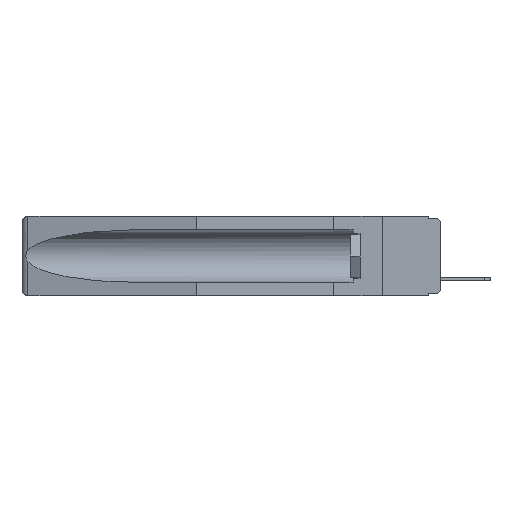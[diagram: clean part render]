
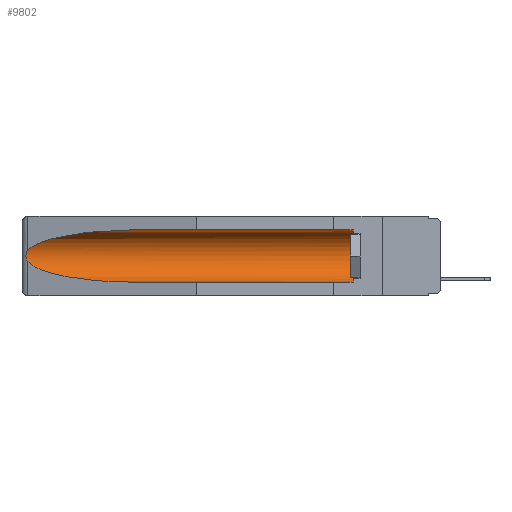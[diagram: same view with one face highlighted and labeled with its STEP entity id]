
A CAD part, left-side view. The second image highlights one B-rep face of the part: STEP entity #9802.
In plain terms, the highlighted cylindrical face has radius 2.857 mm (diameter 5.715 mm), a partial arc.
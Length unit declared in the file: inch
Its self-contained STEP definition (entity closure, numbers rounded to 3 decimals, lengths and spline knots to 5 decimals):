
#357 = VECTOR ( 'NONE', #11340, 39.37008 ) ;
#652 = ORIENTED_EDGE ( 'NONE', *, *, #13948, .F. ) ;
#1512 = CARTESIAN_POINT ( 'NONE',  ( 0.26655, 1.53094, -0.18657 ) ) ;
#1581 = B_SPLINE_CURVE_WITH_KNOTS ( 'NONE', 3,
 ( #2732, #9397, #1680, #13394, #14786, #6887, #8199, #1512, #14873, #12011 ),
 .UNSPECIFIED., .F., .F.,
 ( 4, 2, 2, 2, 4 ),
 ( 0., 0.00029, 0.00058, 0.00087, 0.00117 ),
 .UNSPECIFIED. ) ;
#1680 = CARTESIAN_POINT ( 'NONE',  ( 0.26654, 1.53092, -0.15636 ) ) ;
#2118 = EDGE_CURVE ( 'NONE', #3952, #15262, #4069, .T. ) ;
#2311 = CARTESIAN_POINT ( 'NONE',  ( 0.155, 0.126, -0.1715 ) ) ;
#2732 = CARTESIAN_POINT ( 'NONE',  ( 0.26537, 1.52718, -0.14972 ) ) ;
#3671 = VERTEX_POINT ( 'NONE', #10813 ) ;
#3677 = ORIENTED_EDGE ( 'NONE', *, *, #16923, .T. ) ;
#3952 = VERTEX_POINT ( 'NONE', #11153 ) ;
#4069 =( BOUNDED_CURVE ( )  B_SPLINE_CURVE ( 3, ( #6143, #15267, #11444, #15355 ),
 .UNSPECIFIED., .F., .T. ) 
 B_SPLINE_CURVE_WITH_KNOTS ( ( 4, 4 ),
 ( 0.1948, 1.5708 ),
 .UNSPECIFIED. ) 
 CURVE ( )  GEOMETRIC_REPRESENTATION_ITEM ( )  RATIONAL_B_SPLINE_CURVE ( ( 1., 0.848, 0.848, 1. ) ) 
 REPRESENTATION_ITEM ( '' )  );
#4642 = DIRECTION ( 'NONE',  ( 0., 0., 1. ) ) ;
#4895 = CARTESIAN_POINT ( 'NONE',  ( 0.155, -0.30754, -0.1715 ) ) ;
#4920 = CARTESIAN_POINT ( 'NONE',  ( 0.21114, 1.30732, -0.059 ) ) ;
#5428 =( BOUNDED_CURVE ( )  B_SPLINE_CURVE ( 3, ( #12991, #4920, #10303, #7452 ),
 .UNSPECIFIED., .F., .T. ) 
 B_SPLINE_CURVE_WITH_KNOTS ( ( 4, 4 ),
 ( 4.71239, 6.08839 ),
 .UNSPECIFIED. ) 
 CURVE ( )  GEOMETRIC_REPRESENTATION_ITEM ( )  RATIONAL_B_SPLINE_CURVE ( ( 1., 0.848, 0.848, 1. ) ) 
 REPRESENTATION_ITEM ( '' )  );
#6031 = ORIENTED_EDGE ( 'NONE', *, *, #16534, .T. ) ;
#6135 = ORIENTED_EDGE ( 'NONE', *, *, #2118, .T. ) ;
#6143 = CARTESIAN_POINT ( 'NONE',  ( 0.26537, 1.52718, -0.19328 ) ) ;
#6273 = VERTEX_POINT ( 'NONE', #8053 ) ;
#6887 = CARTESIAN_POINT ( 'NONE',  ( 0.2675, 1.53308, -0.17534 ) ) ;
#7030 = EDGE_LOOP ( 'NONE', ( #6031, #11529, #6135, #652, #3677, #14416 ) ) ;
#7452 = CARTESIAN_POINT ( 'NONE',  ( 0.26537, 1.52718, -0.14972 ) ) ;
#7503 = CARTESIAN_POINT ( 'NONE',  ( 0.155, -0.30754, -0.284 ) ) ;
#8053 = CARTESIAN_POINT ( 'NONE',  ( 0.155, 1.07973, -0.059 ) ) ;
#8199 = CARTESIAN_POINT ( 'NONE',  ( 0.2673, 1.53269, -0.17917 ) ) ;
#9397 = CARTESIAN_POINT ( 'NONE',  ( 0.26597, 1.52961, -0.15275 ) ) ;
#9802 = ADVANCED_FACE ( 'NONE', ( #11234 ), #16543, .F. ) ;
#9959 = CARTESIAN_POINT ( 'NONE',  ( 0.155, -0.30754, -0.059 ) ) ;
#10303 = CARTESIAN_POINT ( 'NONE',  ( 0.25451, 1.48313, -0.09465 ) ) ;
#10427 = VERTEX_POINT ( 'NONE', #13542 ) ;
#10813 = CARTESIAN_POINT ( 'NONE',  ( 0.155, 0.126, -0.284 ) ) ;
#11153 = CARTESIAN_POINT ( 'NONE',  ( 0.26537, 1.52718, -0.19328 ) ) ;
#11234 = FACE_OUTER_BOUND ( 'NONE', #7030, .T. ) ;
#11340 = DIRECTION ( 'NONE',  ( 0., 1., 0. ) ) ;
#11444 = CARTESIAN_POINT ( 'NONE',  ( 0.21114, 1.30732, -0.284 ) ) ;
#11529 = ORIENTED_EDGE ( 'NONE', *, *, #15424, .T. ) ;
#12011 = CARTESIAN_POINT ( 'NONE',  ( 0.26537, 1.52718, -0.19328 ) ) ;
#12796 = DIRECTION ( 'NONE',  ( 0., 1., 0. ) ) ;
#12822 = LINE ( 'NONE', #9959, #357 ) ;
#12969 = DIRECTION ( 'NONE',  ( 0., 0., 1. ) ) ;
#12991 = CARTESIAN_POINT ( 'NONE',  ( 0.155, 1.07973, -0.059 ) ) ;
#13144 = CARTESIAN_POINT ( 'NONE',  ( 0.155, 0.126, -0.059 ) ) ;
#13357 = VECTOR ( 'NONE', #12796, 39.37008 ) ;
#13394 = CARTESIAN_POINT ( 'NONE',  ( 0.2673, 1.5327, -0.16383 ) ) ;
#13542 = CARTESIAN_POINT ( 'NONE',  ( 0.26537, 1.52718, -0.14972 ) ) ;
#13948 = EDGE_CURVE ( 'NONE', #3671, #15262, #15146, .T. ) ;
#14025 = DIRECTION ( 'NONE',  ( 0., -1., 0. ) ) ;
#14416 = ORIENTED_EDGE ( 'NONE', *, *, #14694, .T. ) ;
#14470 = AXIS2_PLACEMENT_3D ( 'NONE', #4895, #15058, #4642 ) ;
#14694 = EDGE_CURVE ( 'NONE', #17107, #6273, #12822, .T. ) ;
#14786 = CARTESIAN_POINT ( 'NONE',  ( 0.2675, 1.53308, -0.16763 ) ) ;
#14873 = CARTESIAN_POINT ( 'NONE',  ( 0.26597, 1.5296, -0.19026 ) ) ;
#15058 = DIRECTION ( 'NONE',  ( 0., 1., 0. ) ) ;
#15146 = LINE ( 'NONE', #7503, #13357 ) ;
#15262 = VERTEX_POINT ( 'NONE', #15929 ) ;
#15267 = CARTESIAN_POINT ( 'NONE',  ( 0.25451, 1.48313, -0.24835 ) ) ;
#15344 = AXIS2_PLACEMENT_3D ( 'NONE', #2311, #14025, #12969 ) ;
#15355 = CARTESIAN_POINT ( 'NONE',  ( 0.155, 1.07973, -0.284 ) ) ;
#15424 = EDGE_CURVE ( 'NONE', #10427, #3952, #1581, .T. ) ;
#15929 = CARTESIAN_POINT ( 'NONE',  ( 0.155, 1.07973, -0.284 ) ) ;
#16534 = EDGE_CURVE ( 'NONE', #6273, #10427, #5428, .T. ) ;
#16543 = CYLINDRICAL_SURFACE ( 'NONE', #14470, 0.1125 ) ;
#16923 = EDGE_CURVE ( 'NONE', #3671, #17107, #17002, .T. ) ;
#17002 = CIRCLE ( 'NONE', #15344, 0.1125 ) ;
#17107 = VERTEX_POINT ( 'NONE', #13144 ) ;
